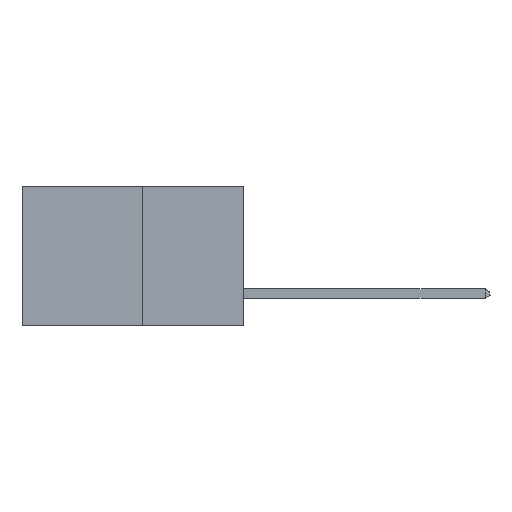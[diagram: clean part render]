
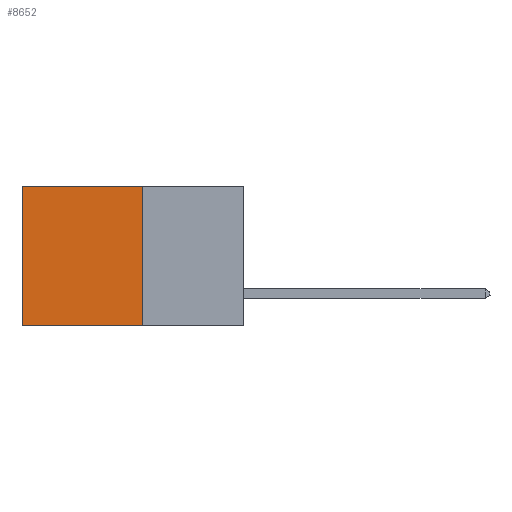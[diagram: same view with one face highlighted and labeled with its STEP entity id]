
A CAD part, left-side view. The second image highlights one B-rep face of the part: STEP entity #8652.
In plain terms, the highlighted planar face has unit normal (-1, 0, 0).
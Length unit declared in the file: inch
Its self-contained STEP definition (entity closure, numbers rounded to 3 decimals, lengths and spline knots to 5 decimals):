
#1550 = DIRECTION ( 'NONE',  ( 0., 1., 0. ) ) ;
#1765 = VECTOR ( 'NONE', #14956, 39.37008 ) ;
#2487 = VERTEX_POINT ( 'NONE', #22270 ) ;
#3011 = ORIENTED_EDGE ( 'NONE', *, *, #5487, .F. ) ;
#4744 = VERTEX_POINT ( 'NONE', #5587 ) ;
#4796 = VECTOR ( 'NONE', #1550, 39.37008 ) ;
#5247 = VERTEX_POINT ( 'NONE', #27451 ) ;
#5487 = EDGE_CURVE ( 'NONE', #2487, #5247, #19484, .T. ) ;
#5587 = CARTESIAN_POINT ( 'NONE',  ( 0.277, 0.59, 0. ) ) ;
#6068 = EDGE_LOOP ( 'NONE', ( #14596, #22687, #3011, #6301 ) ) ;
#6161 = VECTOR ( 'NONE', #15924, 39.37008 ) ;
#6301 = ORIENTED_EDGE ( 'NONE', *, *, #18140, .T. ) ;
#6310 = PLANE ( 'NONE',  #13203 ) ;
#7833 = LINE ( 'NONE', #8159, #1765 ) ;
#8159 = CARTESIAN_POINT ( 'NONE',  ( 0.277, 0.59, -0.37 ) ) ;
#8400 = CARTESIAN_POINT ( 'NONE',  ( 0.277, 0.27, -0.37 ) ) ;
#8652 = ADVANCED_FACE ( 'NONE', ( #13548 ), #6310, .F. ) ;
#10751 = EDGE_CURVE ( 'NONE', #4744, #12001, #7833, .T. ) ;
#10820 = DIRECTION ( 'NONE',  ( 0., 0., -1. ) ) ;
#12001 = VERTEX_POINT ( 'NONE', #14691 ) ;
#12141 = LINE ( 'NONE', #15833, #6161 ) ;
#13203 = AXIS2_PLACEMENT_3D ( 'NONE', #15268, #24294, #10820 ) ;
#13548 = FACE_OUTER_BOUND ( 'NONE', #6068, .T. ) ;
#14596 = ORIENTED_EDGE ( 'NONE', *, *, #10751, .T. ) ;
#14691 = CARTESIAN_POINT ( 'NONE',  ( 0.277, 0.59, -0.37 ) ) ;
#14956 = DIRECTION ( 'NONE',  ( 0., 0., -1. ) ) ;
#15268 = CARTESIAN_POINT ( 'NONE',  ( 0.277, 0.27, -0.37 ) ) ;
#15833 = CARTESIAN_POINT ( 'NONE',  ( 0.277, 0.27, 0. ) ) ;
#15924 = DIRECTION ( 'NONE',  ( 0., 1., 0. ) ) ;
#17479 = DIRECTION ( 'NONE',  ( 0., 0., -1. ) ) ;
#18140 = EDGE_CURVE ( 'NONE', #2487, #4744, #12141, .T. ) ;
#19484 = LINE ( 'NONE', #8400, #24744 ) ;
#22270 = CARTESIAN_POINT ( 'NONE',  ( 0.277, 0.27, 0. ) ) ;
#22687 = ORIENTED_EDGE ( 'NONE', *, *, #26757, .F. ) ;
#23483 = LINE ( 'NONE', #28500, #4796 ) ;
#24294 = DIRECTION ( 'NONE',  ( 1., 0., 0. ) ) ;
#24744 = VECTOR ( 'NONE', #17479, 39.37008 ) ;
#26757 = EDGE_CURVE ( 'NONE', #5247, #12001, #23483, .T. ) ;
#27451 = CARTESIAN_POINT ( 'NONE',  ( 0.277, 0.27, -0.37 ) ) ;
#28500 = CARTESIAN_POINT ( 'NONE',  ( 0.277, 0.27, -0.37 ) ) ;
